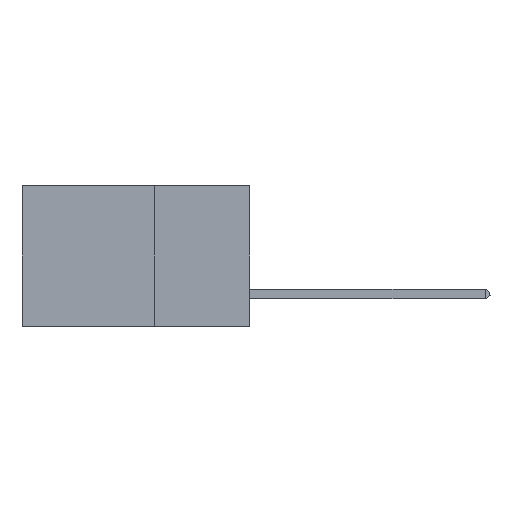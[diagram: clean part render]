
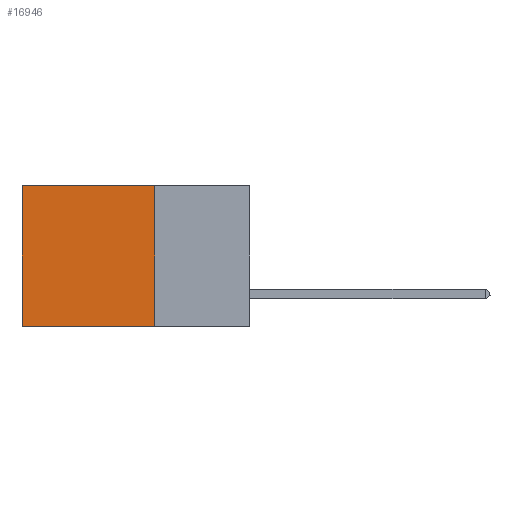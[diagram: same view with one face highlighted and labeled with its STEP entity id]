
A CAD part, left-side view. The second image highlights one B-rep face of the part: STEP entity #16946.
In plain terms, the highlighted planar face has unit normal (-1, 0, 0).
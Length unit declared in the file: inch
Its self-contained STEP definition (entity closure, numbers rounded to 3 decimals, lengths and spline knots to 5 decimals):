
#168 = VECTOR ( 'NONE', #16814, 39.37008 ) ;
#1867 = EDGE_CURVE ( 'NONE', #6629, #17112, #31264, .T. ) ;
#2527 = PLANE ( 'NONE',  #29456 ) ;
#3289 = CARTESIAN_POINT ( 'NONE',  ( 0.2875, 0.25, -0.37 ) ) ;
#3514 = ORIENTED_EDGE ( 'NONE', *, *, #1867, .F. ) ;
#4168 = EDGE_CURVE ( 'NONE', #6629, #20912, #16276, .T. ) ;
#4352 = EDGE_CURVE ( 'NONE', #20912, #6915, #5173, .T. ) ;
#4928 = CARTESIAN_POINT ( 'NONE',  ( 0.2875, 0.25, 0. ) ) ;
#5042 = ORIENTED_EDGE ( 'NONE', *, *, #10628, .F. ) ;
#5173 = LINE ( 'NONE', #6121, #20417 ) ;
#6039 = CARTESIAN_POINT ( 'NONE',  ( 0.2875, 0.6, 0. ) ) ;
#6121 = CARTESIAN_POINT ( 'NONE',  ( 0.2875, 0.6, 0. ) ) ;
#6629 = VERTEX_POINT ( 'NONE', #16507 ) ;
#6915 = VERTEX_POINT ( 'NONE', #30884 ) ;
#9775 = CARTESIAN_POINT ( 'NONE',  ( 0.2875, 0.25, 0. ) ) ;
#9812 = CARTESIAN_POINT ( 'NONE',  ( 0.2875, 0.25, 0. ) ) ;
#10628 = EDGE_CURVE ( 'NONE', #17112, #6915, #13616, .T. ) ;
#12365 = DIRECTION ( 'NONE',  ( 0., 0., -1. ) ) ;
#12680 = EDGE_LOOP ( 'NONE', ( #16003, #5042, #3514, #31308 ) ) ;
#13616 = LINE ( 'NONE', #29765, #20457 ) ;
#14824 = VECTOR ( 'NONE', #21987, 39.37008 ) ;
#15416 = FACE_OUTER_BOUND ( 'NONE', #12680, .T. ) ;
#16003 = ORIENTED_EDGE ( 'NONE', *, *, #4352, .T. ) ;
#16276 = LINE ( 'NONE', #9775, #168 ) ;
#16507 = CARTESIAN_POINT ( 'NONE',  ( 0.2875, 0.25, 0. ) ) ;
#16814 = DIRECTION ( 'NONE',  ( 0., 1., 0. ) ) ;
#16946 = ADVANCED_FACE ( 'NONE', ( #15416 ), #2527, .F. ) ;
#17112 = VERTEX_POINT ( 'NONE', #3289 ) ;
#19508 = DIRECTION ( 'NONE',  ( 1., 0., 0. ) ) ;
#20417 = VECTOR ( 'NONE', #28209, 39.37008 ) ;
#20457 = VECTOR ( 'NONE', #27018, 39.37008 ) ;
#20912 = VERTEX_POINT ( 'NONE', #6039 ) ;
#21987 = DIRECTION ( 'NONE',  ( 0., 0., -1. ) ) ;
#27018 = DIRECTION ( 'NONE',  ( 0., 1., 0. ) ) ;
#28209 = DIRECTION ( 'NONE',  ( 0., 0., -1. ) ) ;
#29456 = AXIS2_PLACEMENT_3D ( 'NONE', #9812, #19508, #12365 ) ;
#29765 = CARTESIAN_POINT ( 'NONE',  ( 0.2875, 0.25, -0.37 ) ) ;
#30884 = CARTESIAN_POINT ( 'NONE',  ( 0.2875, 0.6, -0.37 ) ) ;
#31264 = LINE ( 'NONE', #4928, #14824 ) ;
#31308 = ORIENTED_EDGE ( 'NONE', *, *, #4168, .T. ) ;
